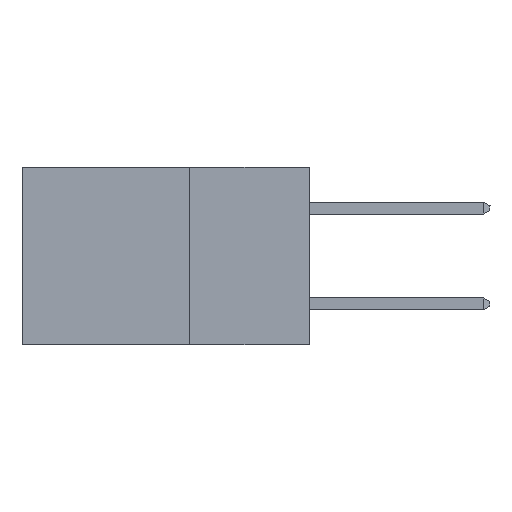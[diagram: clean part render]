
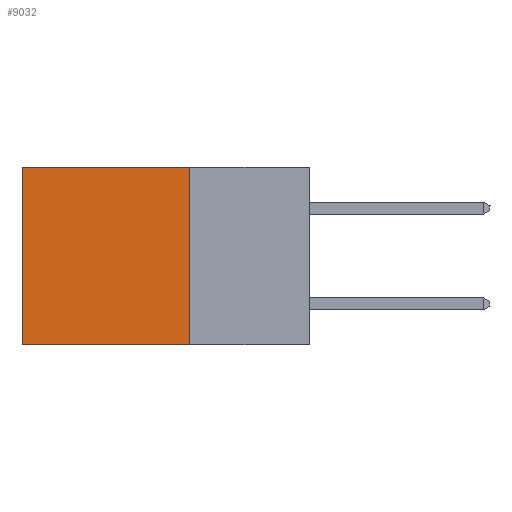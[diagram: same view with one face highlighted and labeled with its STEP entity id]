
A CAD part, left-side view. The second image highlights one B-rep face of the part: STEP entity #9032.
In plain terms, the highlighted planar face has unit normal (-1, 0, 0).
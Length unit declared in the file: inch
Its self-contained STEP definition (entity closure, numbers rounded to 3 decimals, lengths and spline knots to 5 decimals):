
#150 = VERTEX_POINT ( 'NONE', #11359 ) ;
#2189 = FACE_OUTER_BOUND ( 'NONE', #9949, .T. ) ;
#2704 = VECTOR ( 'NONE', #17008, 39.37008 ) ;
#2919 = CARTESIAN_POINT ( 'NONE',  ( 0.2875, 0.25, 0. ) ) ;
#3547 = PLANE ( 'NONE',  #20520 ) ;
#3773 = LINE ( 'NONE', #5310, #8300 ) ;
#3783 = EDGE_CURVE ( 'NONE', #13947, #13048, #13080, .T. ) ;
#4942 = DIRECTION ( 'NONE',  ( 0., 0., -1. ) ) ;
#5310 = CARTESIAN_POINT ( 'NONE',  ( 0.2875, 0.6, 0. ) ) ;
#6379 = VERTEX_POINT ( 'NONE', #6572 ) ;
#6400 = EDGE_CURVE ( 'NONE', #13048, #6379, #3773, .T. ) ;
#6572 = CARTESIAN_POINT ( 'NONE',  ( 0.2875, 0.6, -0.37 ) ) ;
#7695 = VECTOR ( 'NONE', #9871, 39.37008 ) ;
#7736 = CARTESIAN_POINT ( 'NONE',  ( 0.2875, 0.25, 0. ) ) ;
#8300 = VECTOR ( 'NONE', #14777, 39.37008 ) ;
#8632 = EDGE_CURVE ( 'NONE', #13947, #150, #17569, .T. ) ;
#8742 = ORIENTED_EDGE ( 'NONE', *, *, #19889, .F. ) ;
#8893 = CARTESIAN_POINT ( 'NONE',  ( 0.2875, 0.25, 0. ) ) ;
#9032 = ADVANCED_FACE ( 'NONE', ( #2189 ), #3547, .F. ) ;
#9871 = DIRECTION ( 'NONE',  ( 0., 1., 0. ) ) ;
#9949 = EDGE_LOOP ( 'NONE', ( #14315, #8742, #19423, #12262 ) ) ;
#10370 = DIRECTION ( 'NONE',  ( 1., 0., 0. ) ) ;
#10493 = DIRECTION ( 'NONE',  ( 0., 1., 0. ) ) ;
#11359 = CARTESIAN_POINT ( 'NONE',  ( 0.2875, 0.25, -0.37 ) ) ;
#12076 = CARTESIAN_POINT ( 'NONE',  ( 0.2875, 0.25, 0. ) ) ;
#12262 = ORIENTED_EDGE ( 'NONE', *, *, #3783, .T. ) ;
#13048 = VERTEX_POINT ( 'NONE', #16557 ) ;
#13080 = LINE ( 'NONE', #8893, #19060 ) ;
#13947 = VERTEX_POINT ( 'NONE', #2919 ) ;
#14315 = ORIENTED_EDGE ( 'NONE', *, *, #6400, .T. ) ;
#14436 = CARTESIAN_POINT ( 'NONE',  ( 0.2875, 0.25, -0.37 ) ) ;
#14777 = DIRECTION ( 'NONE',  ( 0., 0., -1. ) ) ;
#16557 = CARTESIAN_POINT ( 'NONE',  ( 0.2875, 0.6, 0. ) ) ;
#17008 = DIRECTION ( 'NONE',  ( 0., 0., -1. ) ) ;
#17351 = LINE ( 'NONE', #14436, #7695 ) ;
#17569 = LINE ( 'NONE', #7736, #2704 ) ;
#19060 = VECTOR ( 'NONE', #10493, 39.37008 ) ;
#19423 = ORIENTED_EDGE ( 'NONE', *, *, #8632, .F. ) ;
#19889 = EDGE_CURVE ( 'NONE', #150, #6379, #17351, .T. ) ;
#20520 = AXIS2_PLACEMENT_3D ( 'NONE', #12076, #10370, #4942 ) ;
